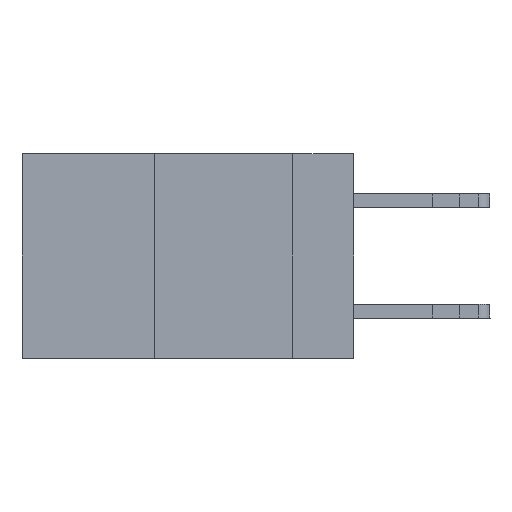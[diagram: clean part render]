
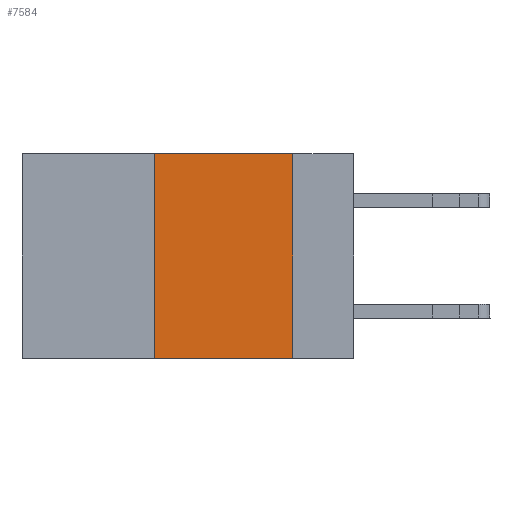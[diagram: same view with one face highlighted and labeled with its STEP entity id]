
A CAD part, left-side view. The second image highlights one B-rep face of the part: STEP entity #7584.
In plain terms, the highlighted planar face has unit normal (-1, 0, 0).
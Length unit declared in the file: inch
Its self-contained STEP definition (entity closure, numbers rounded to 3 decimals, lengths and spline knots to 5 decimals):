
#318 = DIRECTION ( 'NONE',  ( 1., 0., 0. ) ) ;
#513 = VECTOR ( 'NONE', #26069, 39.37008 ) ;
#2986 = CARTESIAN_POINT ( 'NONE',  ( 0., 0.36, -0.37 ) ) ;
#3084 = FACE_OUTER_BOUND ( 'NONE', #20996, .T. ) ;
#3473 = ORIENTED_EDGE ( 'NONE', *, *, #14104, .F. ) ;
#6803 = DIRECTION ( 'NONE',  ( 0., 0., -1. ) ) ;
#7170 = VERTEX_POINT ( 'NONE', #24909 ) ;
#7584 = ADVANCED_FACE ( 'NONE', ( #3084 ), #17425, .F. ) ;
#7650 = LINE ( 'NONE', #13551, #19447 ) ;
#9570 = VECTOR ( 'NONE', #22507, 39.37008 ) ;
#11613 = ORIENTED_EDGE ( 'NONE', *, *, #22660, .T. ) ;
#11874 = LINE ( 'NONE', #14112, #9570 ) ;
#12966 = EDGE_CURVE ( 'NONE', #19298, #18534, #7650, .T. ) ;
#13551 = CARTESIAN_POINT ( 'NONE',  ( 0., 0.36, 0. ) ) ;
#14104 = EDGE_CURVE ( 'NONE', #18534, #7170, #11874, .T. ) ;
#14112 = CARTESIAN_POINT ( 'NONE',  ( 0., 0.6, 0. ) ) ;
#14935 = EDGE_CURVE ( 'NONE', #7170, #15886, #16232, .T. ) ;
#15550 = CARTESIAN_POINT ( 'NONE',  ( 0., 0.11, 0. ) ) ;
#15886 = VERTEX_POINT ( 'NONE', #18004 ) ;
#16232 = LINE ( 'NONE', #15550, #513 ) ;
#16749 = ORIENTED_EDGE ( 'NONE', *, *, #14935, .F. ) ;
#17425 = PLANE ( 'NONE',  #26163 ) ;
#17914 = DIRECTION ( 'NONE',  ( 0., -1., 0. ) ) ;
#18004 = CARTESIAN_POINT ( 'NONE',  ( 0., 0.11, -0.37 ) ) ;
#18534 = VERTEX_POINT ( 'NONE', #26455 ) ;
#19298 = VERTEX_POINT ( 'NONE', #2986 ) ;
#19447 = VECTOR ( 'NONE', #22675, 39.37008 ) ;
#19529 = CARTESIAN_POINT ( 'NONE',  ( 0., 0.6, 0. ) ) ;
#20996 = EDGE_LOOP ( 'NONE', ( #16749, #3473, #26285, #11613 ) ) ;
#21082 = LINE ( 'NONE', #24043, #24998 ) ;
#22507 = DIRECTION ( 'NONE',  ( 0., -1., 0. ) ) ;
#22660 = EDGE_CURVE ( 'NONE', #19298, #15886, #21082, .T. ) ;
#22675 = DIRECTION ( 'NONE',  ( 0., 0., 1. ) ) ;
#24043 = CARTESIAN_POINT ( 'NONE',  ( 0., 0.6, -0.37 ) ) ;
#24909 = CARTESIAN_POINT ( 'NONE',  ( 0., 0.11, 0. ) ) ;
#24998 = VECTOR ( 'NONE', #17914, 39.37008 ) ;
#26069 = DIRECTION ( 'NONE',  ( 0., 0., -1. ) ) ;
#26163 = AXIS2_PLACEMENT_3D ( 'NONE', #19529, #318, #6803 ) ;
#26285 = ORIENTED_EDGE ( 'NONE', *, *, #12966, .F. ) ;
#26455 = CARTESIAN_POINT ( 'NONE',  ( 0., 0.36, 0. ) ) ;
